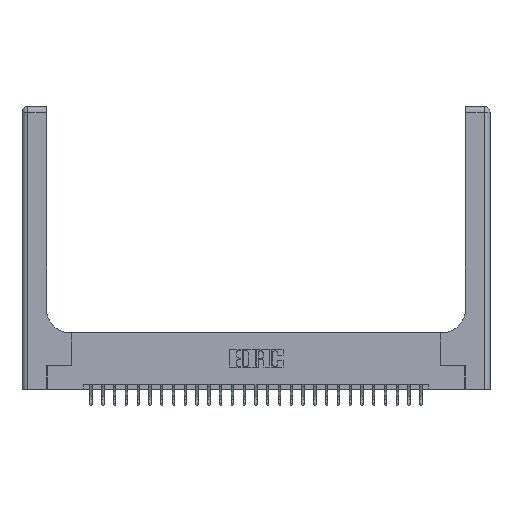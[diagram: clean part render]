
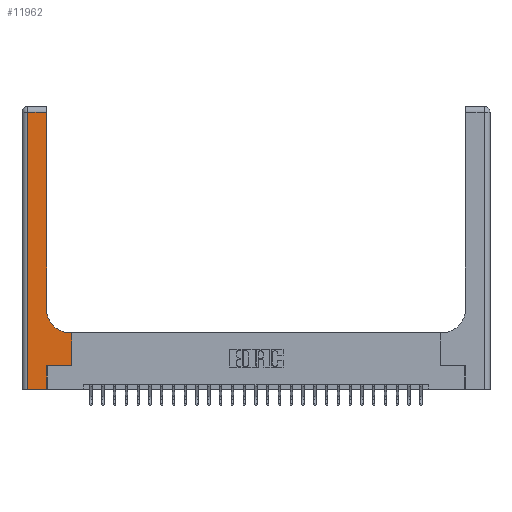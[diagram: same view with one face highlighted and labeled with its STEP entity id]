
A CAD part, top view. The second image highlights one B-rep face of the part: STEP entity #11962.
In plain terms, the highlighted planar face has unit normal (0, 0, 1).
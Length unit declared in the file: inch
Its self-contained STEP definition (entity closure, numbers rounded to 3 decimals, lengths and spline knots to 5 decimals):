
#67 = DIRECTION ( 'NONE',  ( 0., 1., 0. ) ) ;
#316 = VERTEX_POINT ( 'NONE', #5445 ) ;
#453 = LINE ( 'NONE', #12170, #4489 ) ;
#822 = VERTEX_POINT ( 'NONE', #7921 ) ;
#1539 = ORIENTED_EDGE ( 'NONE', *, *, #12671, .T. ) ;
#1792 = EDGE_CURVE ( 'NONE', #11842, #22478, #17811, .T. ) ;
#2427 = CARTESIAN_POINT ( 'NONE',  ( 0.51, 0.6, 0.37 ) ) ;
#2495 = ORIENTED_EDGE ( 'NONE', *, *, #22313, .T. ) ;
#2512 = CARTESIAN_POINT ( 'NONE',  ( 0.06, 3., 0.37 ) ) ;
#2772 = ORIENTED_EDGE ( 'NONE', *, *, #1792, .T. ) ;
#2790 = AXIS2_PLACEMENT_3D ( 'NONE', #20644, #22505, #20291 ) ;
#2885 = ORIENTED_EDGE ( 'NONE', *, *, #7203, .T. ) ;
#3878 = EDGE_CURVE ( 'NONE', #25822, #316, #10123, .T. ) ;
#3914 = FACE_OUTER_BOUND ( 'NONE', #15753, .T. ) ;
#4075 = LINE ( 'NONE', #2512, #8168 ) ;
#4489 = VECTOR ( 'NONE', #67, 39.37008 ) ;
#4716 = AXIS2_PLACEMENT_3D ( 'NONE', #14081, #19855, #23894 ) ;
#5445 = CARTESIAN_POINT ( 'NONE',  ( 0.06, 2.94, 0.37 ) ) ;
#5977 = LINE ( 'NONE', #21036, #17360 ) ;
#7203 = EDGE_CURVE ( 'NONE', #22478, #14572, #7948, .T. ) ;
#7662 = CARTESIAN_POINT ( 'NONE',  ( 0.528, 0.6, 0.37 ) ) ;
#7700 = CARTESIAN_POINT ( 'NONE',  ( 0.26, 0.6, 0.37 ) ) ;
#7921 = CARTESIAN_POINT ( 'NONE',  ( 0.265, 0., 0.37 ) ) ;
#7948 = CIRCLE ( 'NONE', #2790, 0.25 ) ;
#8044 = CARTESIAN_POINT ( 'NONE',  ( 0.06, 0., 0.37 ) ) ;
#8168 = VECTOR ( 'NONE', #24819, 39.37008 ) ;
#8535 = VECTOR ( 'NONE', #24495, 39.37008 ) ;
#9791 = PLANE ( 'NONE',  #4716 ) ;
#10123 = LINE ( 'NONE', #22820, #12296 ) ;
#10647 = DIRECTION ( 'NONE',  ( -1., 0., 0. ) ) ;
#10738 = VERTEX_POINT ( 'NONE', #14052 ) ;
#11243 = DIRECTION ( 'NONE',  ( 0., 1., 0. ) ) ;
#11842 = VERTEX_POINT ( 'NONE', #7662 ) ;
#11962 = ADVANCED_FACE ( 'NONE', ( #3914 ), #9791, .F. ) ;
#12170 = CARTESIAN_POINT ( 'NONE',  ( 0.265, 0., 0.37 ) ) ;
#12296 = VECTOR ( 'NONE', #10647, 39.37008 ) ;
#12671 = EDGE_CURVE ( 'NONE', #15570, #11842, #20798, .T. ) ;
#13945 = DIRECTION ( 'NONE',  ( 1., 0., 0. ) ) ;
#13955 = CARTESIAN_POINT ( 'NONE',  ( 0.528, 0.25, 0.37 ) ) ;
#14052 = CARTESIAN_POINT ( 'NONE',  ( 0.265, 0.25, 0.37 ) ) ;
#14081 = CARTESIAN_POINT ( 'NONE',  ( 0., 3., 0.37 ) ) ;
#14136 = DIRECTION ( 'NONE',  ( 0., 1., 0. ) ) ;
#14335 = CARTESIAN_POINT ( 'NONE',  ( 0., 0., 0.37 ) ) ;
#14572 = VERTEX_POINT ( 'NONE', #25997 ) ;
#14802 = VECTOR ( 'NONE', #14136, 39.37008 ) ;
#15570 = VERTEX_POINT ( 'NONE', #25323 ) ;
#15753 = EDGE_LOOP ( 'NONE', ( #22595, #18322, #21340, #21456, #2495, #16461, #1539, #2772, #2885 ) ) ;
#16461 = ORIENTED_EDGE ( 'NONE', *, *, #25900, .T. ) ;
#16626 = VECTOR ( 'NONE', #13945, 39.37008 ) ;
#17245 = LINE ( 'NONE', #26068, #16626 ) ;
#17360 = VECTOR ( 'NONE', #11243, 39.37008 ) ;
#17811 = LINE ( 'NONE', #7700, #22225 ) ;
#18202 = EDGE_CURVE ( 'NONE', #14572, #25822, #5977, .T. ) ;
#18322 = ORIENTED_EDGE ( 'NONE', *, *, #3878, .T. ) ;
#19855 = DIRECTION ( 'NONE',  ( 0., 0., -1. ) ) ;
#20291 = DIRECTION ( 'NONE',  ( 1., 0., 0. ) ) ;
#20644 = CARTESIAN_POINT ( 'NONE',  ( 0.51, 0.85, 0.37 ) ) ;
#20798 = LINE ( 'NONE', #13955, #14802 ) ;
#20828 = LINE ( 'NONE', #14335, #8535 ) ;
#21036 = CARTESIAN_POINT ( 'NONE',  ( 0.26, 3., 0.37 ) ) ;
#21340 = ORIENTED_EDGE ( 'NONE', *, *, #24240, .T. ) ;
#21456 = ORIENTED_EDGE ( 'NONE', *, *, #23546, .T. ) ;
#22000 = CARTESIAN_POINT ( 'NONE',  ( 0.26, 2.94, 0.37 ) ) ;
#22225 = VECTOR ( 'NONE', #25880, 39.37008 ) ;
#22313 = EDGE_CURVE ( 'NONE', #822, #10738, #453, .T. ) ;
#22478 = VERTEX_POINT ( 'NONE', #2427 ) ;
#22505 = DIRECTION ( 'NONE',  ( 0., 0., -1. ) ) ;
#22595 = ORIENTED_EDGE ( 'NONE', *, *, #18202, .T. ) ;
#22820 = CARTESIAN_POINT ( 'NONE',  ( 0., 2.94, 0.37 ) ) ;
#23546 = EDGE_CURVE ( 'NONE', #24076, #822, #20828, .T. ) ;
#23894 = DIRECTION ( 'NONE',  ( -1., 0., 0. ) ) ;
#24076 = VERTEX_POINT ( 'NONE', #8044 ) ;
#24240 = EDGE_CURVE ( 'NONE', #316, #24076, #4075, .T. ) ;
#24495 = DIRECTION ( 'NONE',  ( 1., 0., 0. ) ) ;
#24819 = DIRECTION ( 'NONE',  ( 0., -1., 0. ) ) ;
#25323 = CARTESIAN_POINT ( 'NONE',  ( 0.528, 0.25, 0.37 ) ) ;
#25822 = VERTEX_POINT ( 'NONE', #22000 ) ;
#25880 = DIRECTION ( 'NONE',  ( -1., 0., 0. ) ) ;
#25900 = EDGE_CURVE ( 'NONE', #10738, #15570, #17245, .T. ) ;
#25997 = CARTESIAN_POINT ( 'NONE',  ( 0.26, 0.85, 0.37 ) ) ;
#26068 = CARTESIAN_POINT ( 'NONE',  ( 0.265, 0.25, 0.37 ) ) ;
